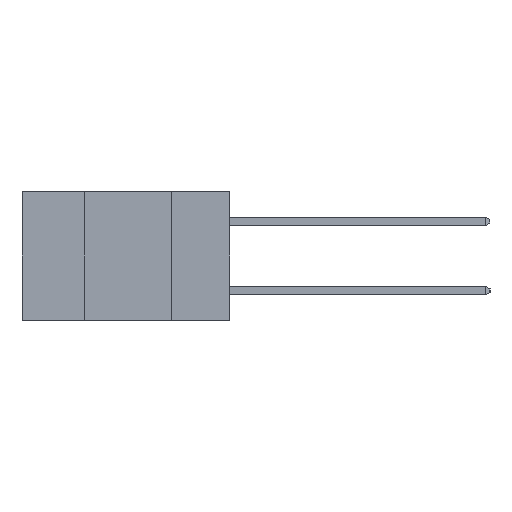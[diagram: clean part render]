
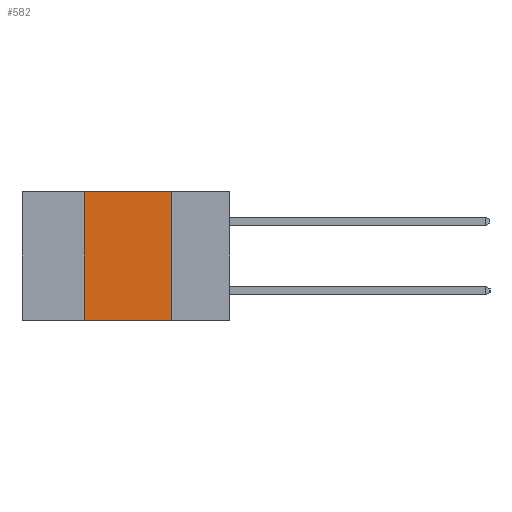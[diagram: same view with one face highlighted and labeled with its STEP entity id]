
A CAD part, left-side view. The second image highlights one B-rep face of the part: STEP entity #582.
In plain terms, the highlighted planar face has unit normal (-1, 0, 0).
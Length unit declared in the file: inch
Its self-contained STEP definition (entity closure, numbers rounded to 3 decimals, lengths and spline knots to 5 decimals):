
#582 = ADVANCED_FACE ( 'NONE', ( #7058 ), #12615, .F. ) ;
#794 = CARTESIAN_POINT ( 'NONE',  ( 0., 0.42, -0.37 ) ) ;
#1331 = DIRECTION ( 'NONE',  ( 1., 0., 0. ) ) ;
#2211 = CARTESIAN_POINT ( 'NONE',  ( 0., 0.17, 0. ) ) ;
#2494 = LINE ( 'NONE', #5887, #17985 ) ;
#3813 = VERTEX_POINT ( 'NONE', #794 ) ;
#5036 = EDGE_CURVE ( 'NONE', #16661, #7639, #2494, .T. ) ;
#5286 = AXIS2_PLACEMENT_3D ( 'NONE', #15125, #1331, #16228 ) ;
#5412 = VECTOR ( 'NONE', #9742, 39.37008 ) ;
#5887 = CARTESIAN_POINT ( 'NONE',  ( 0., 0.6, 0. ) ) ;
#6089 = CARTESIAN_POINT ( 'NONE',  ( 0., 0.17, -0.37 ) ) ;
#6965 = CARTESIAN_POINT ( 'NONE',  ( 0., 0.17, -0.37 ) ) ;
#7058 = FACE_OUTER_BOUND ( 'NONE', #16992, .T. ) ;
#7475 = VECTOR ( 'NONE', #17203, 39.37008 ) ;
#7639 = VERTEX_POINT ( 'NONE', #2211 ) ;
#8862 = DIRECTION ( 'NONE',  ( 0., -1., 0. ) ) ;
#9742 = DIRECTION ( 'NONE',  ( 0., 0., 1. ) ) ;
#10683 = VECTOR ( 'NONE', #12946, 39.37008 ) ;
#10874 = ORIENTED_EDGE ( 'NONE', *, *, #13356, .F. ) ;
#11412 = EDGE_CURVE ( 'NONE', #3813, #14329, #15052, .T. ) ;
#11481 = CARTESIAN_POINT ( 'NONE',  ( 0., 0.6, -0.37 ) ) ;
#11801 = ORIENTED_EDGE ( 'NONE', *, *, #15981, .F. ) ;
#12615 = PLANE ( 'NONE',  #5286 ) ;
#12946 = DIRECTION ( 'NONE',  ( 0., -1., 0. ) ) ;
#13356 = EDGE_CURVE ( 'NONE', #3813, #16661, #17238, .T. ) ;
#14329 = VERTEX_POINT ( 'NONE', #6089 ) ;
#14333 = ORIENTED_EDGE ( 'NONE', *, *, #11412, .T. ) ;
#14355 = LINE ( 'NONE', #6965, #7475 ) ;
#15052 = LINE ( 'NONE', #11481, #10683 ) ;
#15125 = CARTESIAN_POINT ( 'NONE',  ( 0., 0.6, 0. ) ) ;
#15249 = ORIENTED_EDGE ( 'NONE', *, *, #5036, .F. ) ;
#15981 = EDGE_CURVE ( 'NONE', #7639, #14329, #14355, .T. ) ;
#16228 = DIRECTION ( 'NONE',  ( 0., 0., -1. ) ) ;
#16661 = VERTEX_POINT ( 'NONE', #17178 ) ;
#16992 = EDGE_LOOP ( 'NONE', ( #11801, #15249, #10874, #14333 ) ) ;
#17110 = CARTESIAN_POINT ( 'NONE',  ( 0., 0.42, -0.37 ) ) ;
#17178 = CARTESIAN_POINT ( 'NONE',  ( 0., 0.42, 0. ) ) ;
#17203 = DIRECTION ( 'NONE',  ( 0., 0., -1. ) ) ;
#17238 = LINE ( 'NONE', #17110, #5412 ) ;
#17985 = VECTOR ( 'NONE', #8862, 39.37008 ) ;
